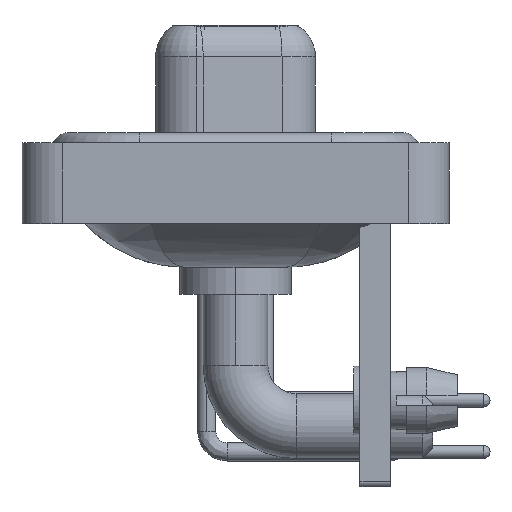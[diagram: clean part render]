
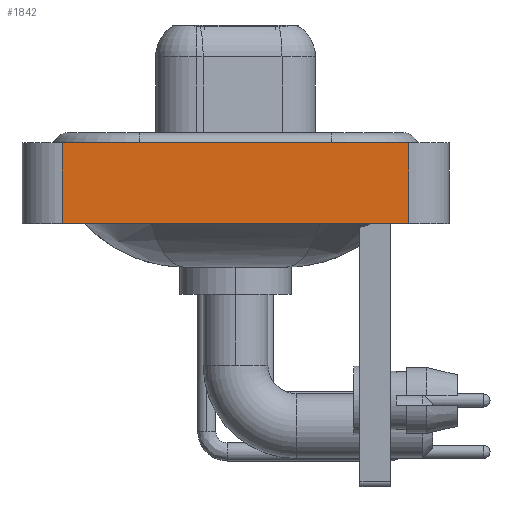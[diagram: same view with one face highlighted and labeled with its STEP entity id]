
A CAD part, left-side view. The second image highlights one B-rep face of the part: STEP entity #1842.
In plain terms, the highlighted planar face has unit normal (-1, 0, 0).
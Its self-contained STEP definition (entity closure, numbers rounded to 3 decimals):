
#99 = CARTESIAN_POINT ( 'NONE',  ( -7.3, -8.55, -3.6 ) ) ;
#138 = ORIENTED_EDGE ( 'NONE', *, *, #19999, .F. ) ;
#248 = CARTESIAN_POINT ( 'NONE',  ( -7.3, 8.55, -3.6 ) ) ;
#1842 = ADVANCED_FACE ( 'NONE', ( #13794 ), #6365, .T. ) ;
#2018 = EDGE_CURVE ( 'NONE', #9948, #9713, #7069, .T. ) ;
#2791 = VERTEX_POINT ( 'NONE', #22955 ) ;
#3251 = CARTESIAN_POINT ( 'NONE',  ( -7.3, -8.55, 0.4 ) ) ;
#3484 = VECTOR ( 'NONE', #5565, 1000. ) ;
#3497 = LINE ( 'NONE', #248, #13849 ) ;
#3536 = EDGE_CURVE ( 'NONE', #9713, #5198, #13773, .T. ) ;
#4485 = CARTESIAN_POINT ( 'NONE',  ( -7.3, -8.55, -3.6 ) ) ;
#4835 = DIRECTION ( 'NONE',  ( 0., 0., 1. ) ) ;
#4935 = ORIENTED_EDGE ( 'NONE', *, *, #2018, .T. ) ;
#5198 = VERTEX_POINT ( 'NONE', #3251 ) ;
#5565 = DIRECTION ( 'NONE',  ( 0., -1., 0. ) ) ;
#6365 = PLANE ( 'NONE',  #6443 ) ;
#6443 = AXIS2_PLACEMENT_3D ( 'NONE', #22199, #20905, #6482 ) ;
#6482 = DIRECTION ( 'NONE',  ( 0., 0., 1. ) ) ;
#7069 = LINE ( 'NONE', #99, #3484 ) ;
#9713 = VERTEX_POINT ( 'NONE', #15295 ) ;
#9948 = VERTEX_POINT ( 'NONE', #17858 ) ;
#13323 = EDGE_LOOP ( 'NONE', ( #15506, #138, #16770, #4935 ) ) ;
#13773 = LINE ( 'NONE', #4485, #15798 ) ;
#13794 = FACE_OUTER_BOUND ( 'NONE', #13323, .T. ) ;
#13849 = VECTOR ( 'NONE', #18018, 1000. ) ;
#15295 = CARTESIAN_POINT ( 'NONE',  ( -7.3, -8.55, -3.6 ) ) ;
#15506 = ORIENTED_EDGE ( 'NONE', *, *, #3536, .T. ) ;
#15798 = VECTOR ( 'NONE', #4835, 1000. ) ;
#16312 = DIRECTION ( 'NONE',  ( 0., -1., 0. ) ) ;
#16525 = LINE ( 'NONE', #20037, #20736 ) ;
#16770 = ORIENTED_EDGE ( 'NONE', *, *, #18182, .F. ) ;
#17858 = CARTESIAN_POINT ( 'NONE',  ( -7.3, 8.55, -3.6 ) ) ;
#18018 = DIRECTION ( 'NONE',  ( 0., 0., 1. ) ) ;
#18182 = EDGE_CURVE ( 'NONE', #9948, #2791, #3497, .T. ) ;
#19999 = EDGE_CURVE ( 'NONE', #2791, #5198, #16525, .T. ) ;
#20037 = CARTESIAN_POINT ( 'NONE',  ( -7.3, -8.55, 0.4 ) ) ;
#20736 = VECTOR ( 'NONE', #16312, 1000. ) ;
#20905 = DIRECTION ( 'NONE',  ( -1., 0., 0. ) ) ;
#22199 = CARTESIAN_POINT ( 'NONE',  ( -7.3, -8.55, -3.6 ) ) ;
#22955 = CARTESIAN_POINT ( 'NONE',  ( -7.3, 8.55, 0.4 ) ) ;
